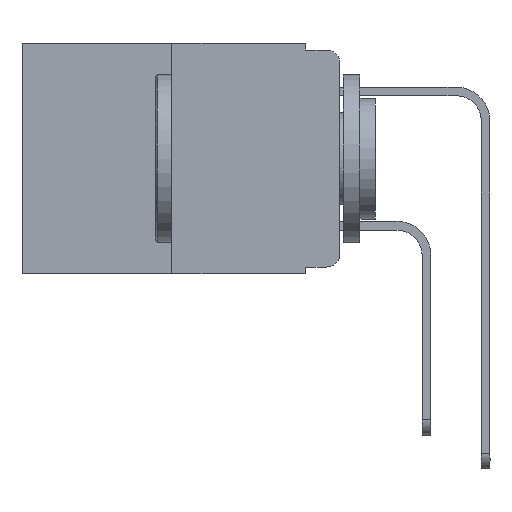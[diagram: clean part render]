
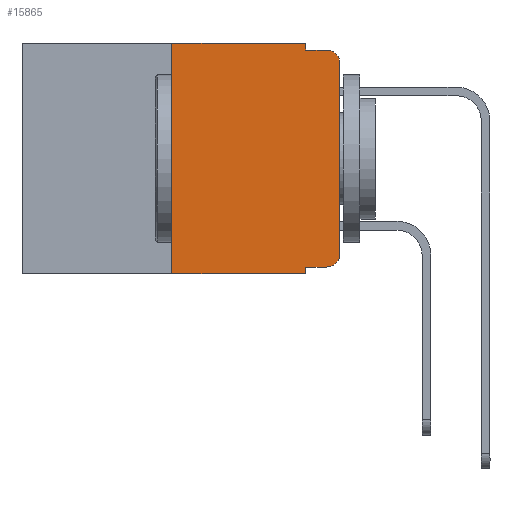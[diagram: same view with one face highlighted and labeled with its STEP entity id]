
A CAD part, left-side view. The second image highlights one B-rep face of the part: STEP entity #15865.
In plain terms, the highlighted planar face has unit normal (-1, 0, 0).
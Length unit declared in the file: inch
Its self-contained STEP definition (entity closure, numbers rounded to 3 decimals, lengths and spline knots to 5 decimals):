
#63 = VERTEX_POINT ( 'NONE', #12963 ) ;
#121 = VERTEX_POINT ( 'NONE', #16251 ) ;
#503 = CARTESIAN_POINT ( 'NONE',  ( 0., 0.02, -0.01 ) ) ;
#545 = CARTESIAN_POINT ( 'NONE',  ( 0., 0.051, -0.343 ) ) ;
#858 = CARTESIAN_POINT ( 'NONE',  ( 0., 0.473, -0.343 ) ) ;
#1083 = VECTOR ( 'NONE', #6788, 39.37008 ) ;
#1514 = VECTOR ( 'NONE', #17692, 39.37008 ) ;
#1670 = EDGE_CURVE ( 'NONE', #63, #1828, #16770, .T. ) ;
#1828 = VERTEX_POINT ( 'NONE', #12881 ) ;
#1999 = VECTOR ( 'NONE', #4646, 39.37008 ) ;
#2464 = DIRECTION ( 'NONE',  ( -1., 0., 0. ) ) ;
#2817 = DIRECTION ( 'NONE',  ( 1., 0., 0. ) ) ;
#3363 = VERTEX_POINT ( 'NONE', #4148 ) ;
#3427 = VECTOR ( 'NONE', #3774, 39.37008 ) ;
#3432 = DIRECTION ( 'NONE',  ( 0., 0., -1. ) ) ;
#3503 = ORIENTED_EDGE ( 'NONE', *, *, #6693, .T. ) ;
#3774 = DIRECTION ( 'NONE',  ( 0., -1., 0. ) ) ;
#3873 = CARTESIAN_POINT ( 'NONE',  ( 0., 0.051, -0.333 ) ) ;
#4148 = CARTESIAN_POINT ( 'NONE',  ( 0., 0., -0.03 ) ) ;
#4162 = LINE ( 'NONE', #3873, #3427 ) ;
#4210 = DIRECTION ( 'NONE',  ( 0., 0., -1. ) ) ;
#4515 = LINE ( 'NONE', #5871, #16084 ) ;
#4646 = DIRECTION ( 'NONE',  ( 0., 0., 1. ) ) ;
#5344 = EDGE_CURVE ( 'NONE', #5354, #17135, #11852, .T. ) ;
#5354 = VERTEX_POINT ( 'NONE', #15742 ) ;
#5493 = ORIENTED_EDGE ( 'NONE', *, *, #5344, .T. ) ;
#5563 = CARTESIAN_POINT ( 'NONE',  ( 0., 0.051, 0. ) ) ;
#5590 = EDGE_CURVE ( 'NONE', #121, #12124, #17505, .T. ) ;
#5614 = VERTEX_POINT ( 'NONE', #5563 ) ;
#5666 = CARTESIAN_POINT ( 'NONE',  ( 0., 0.051, -0.01 ) ) ;
#5871 = CARTESIAN_POINT ( 'NONE',  ( 0., 0.051, -0.01 ) ) ;
#5916 = CARTESIAN_POINT ( 'NONE',  ( 0., 0., -0.313 ) ) ;
#5969 = ORIENTED_EDGE ( 'NONE', *, *, #1670, .F. ) ;
#6267 = ORIENTED_EDGE ( 'NONE', *, *, #10488, .T. ) ;
#6693 = EDGE_CURVE ( 'NONE', #3363, #15095, #17914, .T. ) ;
#6788 = DIRECTION ( 'NONE',  ( 0., -1., 0. ) ) ;
#7414 = CARTESIAN_POINT ( 'NONE',  ( 0., 0.051, 0. ) ) ;
#7477 = PLANE ( 'NONE',  #14765 ) ;
#7711 = ORIENTED_EDGE ( 'NONE', *, *, #11896, .T. ) ;
#7944 = DIRECTION ( 'NONE',  ( 0., 0., 1. ) ) ;
#8281 = CARTESIAN_POINT ( 'NONE',  ( 0., 0.051, 0. ) ) ;
#8704 = EDGE_CURVE ( 'NONE', #1828, #5614, #11760, .T. ) ;
#8869 = EDGE_LOOP ( 'NONE', ( #7711, #3503, #17498, #9556, #18910, #5969, #9697, #13485, #6267, #5493 ) ) ;
#9120 = FACE_OUTER_BOUND ( 'NONE', #8869, .T. ) ;
#9265 = DIRECTION ( 'NONE',  ( -1., 0., 0. ) ) ;
#9493 = CARTESIAN_POINT ( 'NONE',  ( 0., 0.25, 0. ) ) ;
#9556 = ORIENTED_EDGE ( 'NONE', *, *, #9996, .F. ) ;
#9697 = ORIENTED_EDGE ( 'NONE', *, *, #11847, .T. ) ;
#9996 = EDGE_CURVE ( 'NONE', #5614, #11595, #18738, .T. ) ;
#10052 = CARTESIAN_POINT ( 'NONE',  ( 0., 0.02, -0.03 ) ) ;
#10316 = CARTESIAN_POINT ( 'NONE',  ( 0., 0.473, 0. ) ) ;
#10488 = EDGE_CURVE ( 'NONE', #121, #5354, #4162, .T. ) ;
#10535 = DIRECTION ( 'NONE',  ( 0., -1., 0. ) ) ;
#11595 = VERTEX_POINT ( 'NONE', #5666 ) ;
#11648 = CARTESIAN_POINT ( 'NONE',  ( 0., 0.473, 0. ) ) ;
#11760 = LINE ( 'NONE', #10316, #1514 ) ;
#11826 = LINE ( 'NONE', #15003, #1999 ) ;
#11847 = EDGE_CURVE ( 'NONE', #63, #12124, #17560, .T. ) ;
#11852 = CIRCLE ( 'NONE', #18050, 0.02 ) ;
#11896 = EDGE_CURVE ( 'NONE', #17135, #3363, #11826, .T. ) ;
#12124 = VERTEX_POINT ( 'NONE', #545 ) ;
#12881 = CARTESIAN_POINT ( 'NONE',  ( 0., 0.25, 0. ) ) ;
#12963 = CARTESIAN_POINT ( 'NONE',  ( 0., 0.25, -0.343 ) ) ;
#13020 = DIRECTION ( 'NONE',  ( 0., 0., -1. ) ) ;
#13485 = ORIENTED_EDGE ( 'NONE', *, *, #5590, .F. ) ;
#14765 = AXIS2_PLACEMENT_3D ( 'NONE', #11648, #2817, #15014 ) ;
#14794 = AXIS2_PLACEMENT_3D ( 'NONE', #10052, #2464, #15942 ) ;
#15003 = CARTESIAN_POINT ( 'NONE',  ( 0., 0., 0. ) ) ;
#15014 = DIRECTION ( 'NONE',  ( 0., 0., -1. ) ) ;
#15095 = VERTEX_POINT ( 'NONE', #503 ) ;
#15742 = CARTESIAN_POINT ( 'NONE',  ( 0., 0.02, -0.333 ) ) ;
#15865 = ADVANCED_FACE ( 'NONE', ( #9120 ), #7477, .F. ) ;
#15942 = DIRECTION ( 'NONE',  ( 0., 0., -1. ) ) ;
#16084 = VECTOR ( 'NONE', #10535, 39.37008 ) ;
#16251 = CARTESIAN_POINT ( 'NONE',  ( 0., 0.051, -0.333 ) ) ;
#16634 = VECTOR ( 'NONE', #4210, 39.37008 ) ;
#16770 = LINE ( 'NONE', #9493, #18912 ) ;
#17135 = VERTEX_POINT ( 'NONE', #5916 ) ;
#17369 = VECTOR ( 'NONE', #13020, 39.37008 ) ;
#17498 = ORIENTED_EDGE ( 'NONE', *, *, #17946, .F. ) ;
#17505 = LINE ( 'NONE', #7414, #16634 ) ;
#17560 = LINE ( 'NONE', #858, #1083 ) ;
#17692 = DIRECTION ( 'NONE',  ( 0., -1., 0. ) ) ;
#17914 = CIRCLE ( 'NONE', #14794, 0.02 ) ;
#17946 = EDGE_CURVE ( 'NONE', #11595, #15095, #4515, .T. ) ;
#18050 = AXIS2_PLACEMENT_3D ( 'NONE', #18092, #9265, #3432 ) ;
#18092 = CARTESIAN_POINT ( 'NONE',  ( 0., 0.02, -0.313 ) ) ;
#18738 = LINE ( 'NONE', #8281, #17369 ) ;
#18910 = ORIENTED_EDGE ( 'NONE', *, *, #8704, .F. ) ;
#18912 = VECTOR ( 'NONE', #7944, 39.37008 ) ;
